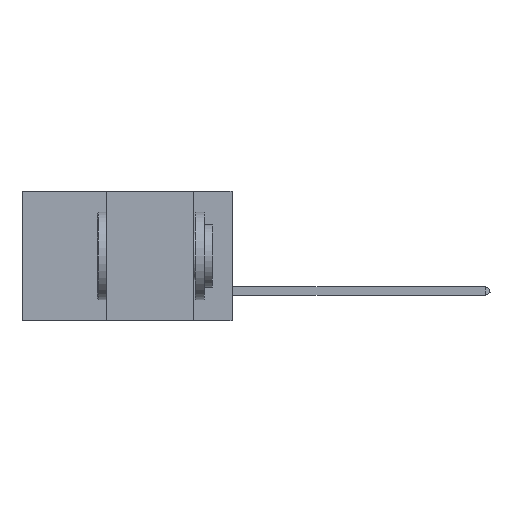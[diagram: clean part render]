
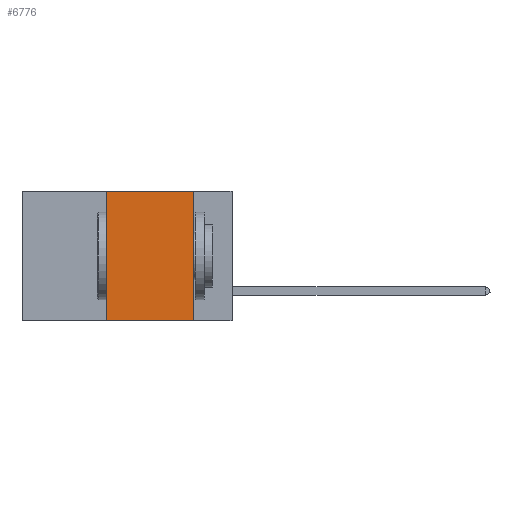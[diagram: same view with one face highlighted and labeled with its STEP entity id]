
A CAD part, left-side view. The second image highlights one B-rep face of the part: STEP entity #6776.
In plain terms, the highlighted planar face has unit normal (-1, 0, 0).
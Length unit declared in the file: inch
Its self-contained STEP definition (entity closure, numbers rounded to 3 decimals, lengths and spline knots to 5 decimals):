
#197 = LINE ( 'NONE', #4050, #805 ) ;
#483 = EDGE_CURVE ( 'NONE', #5421, #2948, #7813, .T. ) ;
#570 = DIRECTION ( 'NONE',  ( 1., 0., 0. ) ) ;
#724 = CARTESIAN_POINT ( 'NONE',  ( 0., 0.11, 0. ) ) ;
#805 = VECTOR ( 'NONE', #3275, 39.37008 ) ;
#819 = LINE ( 'NONE', #4650, #6602 ) ;
#1054 = EDGE_LOOP ( 'NONE', ( #9246, #4048, #7035, #10084 ) ) ;
#1125 = VERTEX_POINT ( 'NONE', #6838 ) ;
#2194 = VECTOR ( 'NONE', #4668, 39.37008 ) ;
#2948 = VERTEX_POINT ( 'NONE', #6813 ) ;
#3275 = DIRECTION ( 'NONE',  ( 0., -1., 0. ) ) ;
#4048 = ORIENTED_EDGE ( 'NONE', *, *, #4426, .F. ) ;
#4050 = CARTESIAN_POINT ( 'NONE',  ( 0., 0.6, 0. ) ) ;
#4181 = FACE_OUTER_BOUND ( 'NONE', #1054, .T. ) ;
#4328 = LINE ( 'NONE', #724, #2194 ) ;
#4426 = EDGE_CURVE ( 'NONE', #2948, #1125, #197, .T. ) ;
#4650 = CARTESIAN_POINT ( 'NONE',  ( 0., 0.6, -0.37 ) ) ;
#4668 = DIRECTION ( 'NONE',  ( 0., 0., -1. ) ) ;
#4941 = CARTESIAN_POINT ( 'NONE',  ( 0., 0.36, -0.37 ) ) ;
#5289 = CARTESIAN_POINT ( 'NONE',  ( 0., 0.6, 0. ) ) ;
#5421 = VERTEX_POINT ( 'NONE', #4941 ) ;
#5610 = DIRECTION ( 'NONE',  ( 0., -1., 0. ) ) ;
#5707 = VECTOR ( 'NONE', #6715, 39.37008 ) ;
#6085 = DIRECTION ( 'NONE',  ( 0., 0., -1. ) ) ;
#6143 = VERTEX_POINT ( 'NONE', #7591 ) ;
#6297 = AXIS2_PLACEMENT_3D ( 'NONE', #5289, #570, #6085 ) ;
#6354 = EDGE_CURVE ( 'NONE', #1125, #6143, #4328, .T. ) ;
#6602 = VECTOR ( 'NONE', #5610, 39.37008 ) ;
#6715 = DIRECTION ( 'NONE',  ( 0., 0., 1. ) ) ;
#6776 = ADVANCED_FACE ( 'NONE', ( #4181 ), #8604, .F. ) ;
#6813 = CARTESIAN_POINT ( 'NONE',  ( 0., 0.36, 0. ) ) ;
#6838 = CARTESIAN_POINT ( 'NONE',  ( 0., 0.11, 0. ) ) ;
#6862 = EDGE_CURVE ( 'NONE', #5421, #6143, #819, .T. ) ;
#7035 = ORIENTED_EDGE ( 'NONE', *, *, #483, .F. ) ;
#7591 = CARTESIAN_POINT ( 'NONE',  ( 0., 0.11, -0.37 ) ) ;
#7813 = LINE ( 'NONE', #9916, #5707 ) ;
#8604 = PLANE ( 'NONE',  #6297 ) ;
#9246 = ORIENTED_EDGE ( 'NONE', *, *, #6354, .F. ) ;
#9916 = CARTESIAN_POINT ( 'NONE',  ( 0., 0.36, 0. ) ) ;
#10084 = ORIENTED_EDGE ( 'NONE', *, *, #6862, .T. ) ;
